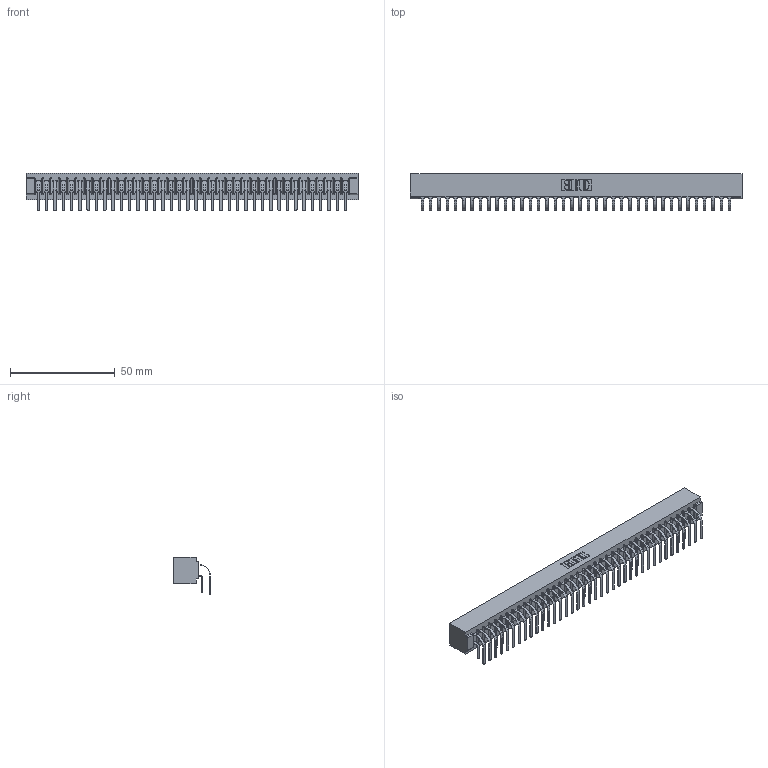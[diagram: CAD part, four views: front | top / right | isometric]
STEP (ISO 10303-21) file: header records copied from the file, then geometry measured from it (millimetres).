
FILE_DESCRIPTION (( 'STEP AP203' ), '1' );
FILE_NAME ('307-076-459-201.STEP', '2022-07-07T19:04:10', ( '' ), ( '' ), 'SwSTEP 2.0', 'SolidWorks 2020', '' );
FILE_SCHEMA (( 'CONFIG_CONTROL_DESIGN' ));
Length unit declared in the file: inch
Products named in the file (4): 307 Part_No Mounting Lugs; 307-290-001_558 559 - 1 (Single); 307-076-459-201; 307-290-001_559 - 2 (Single)
Assembly tree (77 placements, depth 2):
  307-076-459-201
    307 Part_No Mounting Lugs
    307-290-001_558 559 - 1 (Single)  x38
    307-290-001_559 - 2 (Single)  x38
Bounding box: 158.45 x 17.51 x 18.07 mm (x, y, z)
Volume: 17653.8 mm3; surface area: 23463.2 mm2
Topology: 77 solids, 77 shells, 3949 faces, 11091 edges, 7186 vertices
Faces by surface type: plane 2574, cylinder 1297, sphere 78
Entity records: 35455 total; most frequent: CARTESIAN_POINT 5800, ORIENTED_EDGE 5746, DIRECTION 5681, EDGE_CURVE 2873, VECTOR 2203, LINE 2203, VERTEX_POINT 1858, AXIS2_PLACEMENT_3D 1739
